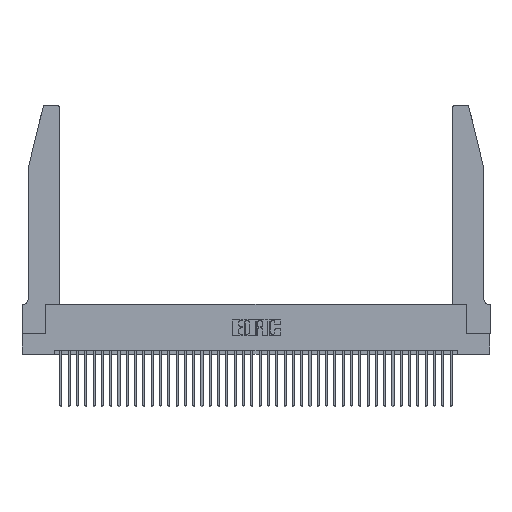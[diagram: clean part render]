
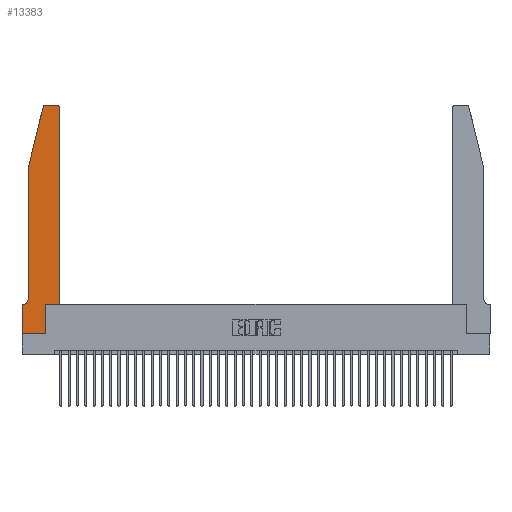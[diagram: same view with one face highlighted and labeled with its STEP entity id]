
A CAD part, top view. The second image highlights one B-rep face of the part: STEP entity #13383.
In plain terms, the highlighted planar face has unit normal (0, 0, 1).
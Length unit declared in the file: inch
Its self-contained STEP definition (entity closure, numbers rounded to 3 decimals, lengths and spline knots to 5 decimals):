
#378 = ORIENTED_EDGE ( 'NONE', *, *, #773, .T. ) ;
#773 = EDGE_CURVE ( 'NONE', #3050, #33618, #16278, .T. ) ;
#1754 = DIRECTION ( 'NONE',  ( -0.239, -0.971, 0. ) ) ;
#2519 = CARTESIAN_POINT ( 'NONE',  ( 0.0755, 2., 0.37 ) ) ;
#2624 = EDGE_CURVE ( 'NONE', #14654, #20736, #34224, .T. ) ;
#2860 = VERTEX_POINT ( 'NONE', #2519 ) ;
#3050 = VERTEX_POINT ( 'NONE', #29282 ) ;
#5523 = DIRECTION ( 'NONE',  ( 0., 0., 1. ) ) ;
#5721 = DIRECTION ( 'NONE',  ( 0., 0., 1. ) ) ;
#5935 = VERTEX_POINT ( 'NONE', #39529 ) ;
#6006 = AXIS2_PLACEMENT_3D ( 'NONE', #24862, #5721, #28077 ) ;
#6922 = ORIENTED_EDGE ( 'NONE', *, *, #25436, .T. ) ;
#7290 = CARTESIAN_POINT ( 'NONE',  ( 0.25487, 2.72718, 0.37 ) ) ;
#8300 = CARTESIAN_POINT ( 'NONE',  ( 0.4505, 0.35, 0.37 ) ) ;
#8853 = EDGE_CURVE ( 'NONE', #40166, #2860, #13556, .T. ) ;
#8968 = VERTEX_POINT ( 'NONE', #15034 ) ;
#9533 = CIRCLE ( 'NONE', #31428, 0.07 ) ;
#9796 = CARTESIAN_POINT ( 'NONE',  ( 0.2865, 0., 0.37 ) ) ;
#9949 = ORIENTED_EDGE ( 'NONE', *, *, #37876, .T. ) ;
#10384 = CARTESIAN_POINT ( 'NONE',  ( 0., 0., 0.37 ) ) ;
#10507 = FACE_OUTER_BOUND ( 'NONE', #39377, .T. ) ;
#10525 = DIRECTION ( 'NONE',  ( 0., 0., -1. ) ) ;
#10629 = CARTESIAN_POINT ( 'NONE',  ( 0.0055, 0.35, 0.37 ) ) ;
#10643 = DIRECTION ( 'NONE',  ( 1., 0., 0. ) ) ;
#10879 = VECTOR ( 'NONE', #37128, 39.37008 ) ;
#11299 = CARTESIAN_POINT ( 'NONE',  ( 0.2865, 0.35, 0.37 ) ) ;
#11422 = CARTESIAN_POINT ( 'NONE',  ( 0., 0., 0.37 ) ) ;
#11469 = ORIENTED_EDGE ( 'NONE', *, *, #29979, .T. ) ;
#12516 = AXIS2_PLACEMENT_3D ( 'NONE', #24664, #5523, #27863 ) ;
#13049 = VECTOR ( 'NONE', #33979, 39.37008 ) ;
#13055 = CIRCLE ( 'NONE', #6006, 0.03 ) ;
#13204 = VERTEX_POINT ( 'NONE', #24292 ) ;
#13383 = ADVANCED_FACE ( 'NONE', ( #10507 ), #31599, .T. ) ;
#13391 = VECTOR ( 'NONE', #10643, 39.37008 ) ;
#13556 = LINE ( 'NONE', #14614, #29543 ) ;
#14490 = ORIENTED_EDGE ( 'NONE', *, *, #14799, .T. ) ;
#14614 = CARTESIAN_POINT ( 'NONE',  ( 0.0755, 2., 0.37 ) ) ;
#14654 = VERTEX_POINT ( 'NONE', #9796 ) ;
#14799 = EDGE_CURVE ( 'NONE', #20736, #5935, #16878, .T. ) ;
#15034 = CARTESIAN_POINT ( 'NONE',  ( 0.284, 2.75, 0.37 ) ) ;
#16278 = CIRCLE ( 'NONE', #12516, 0.03 ) ;
#16878 = LINE ( 'NONE', #26118, #41525 ) ;
#16894 = CARTESIAN_POINT ( 'NONE',  ( 0.0755, 0.35, 0.37 ) ) ;
#17439 = ORIENTED_EDGE ( 'NONE', *, *, #27368, .T. ) ;
#17951 = CARTESIAN_POINT ( 'NONE',  ( 0.0755, 2., 0.37 ) ) ;
#18715 = AXIS2_PLACEMENT_3D ( 'NONE', #34753, #38128, #18847 ) ;
#18847 = DIRECTION ( 'NONE',  ( 1., 0., 0. ) ) ;
#19014 = CARTESIAN_POINT ( 'NONE',  ( 0.4205, 2.75, 0.37 ) ) ;
#20403 = EDGE_CURVE ( 'NONE', #5935, #3050, #34361, .T. ) ;
#20440 = ORIENTED_EDGE ( 'NONE', *, *, #38252, .T. ) ;
#20695 = VERTEX_POINT ( 'NONE', #22513 ) ;
#20736 = VERTEX_POINT ( 'NONE', #39027 ) ;
#21429 = DIRECTION ( 'NONE',  ( 0., 1., 0. ) ) ;
#21852 = LINE ( 'NONE', #32798, #13391 ) ;
#22513 = CARTESIAN_POINT ( 'NONE',  ( 0., 0.35, 0.37 ) ) ;
#23695 = VECTOR ( 'NONE', #30271, 39.37008 ) ;
#23969 = ORIENTED_EDGE ( 'NONE', *, *, #20403, .T. ) ;
#24292 = CARTESIAN_POINT ( 'NONE',  ( 0.0755, 0.42, 0.37 ) ) ;
#24664 = CARTESIAN_POINT ( 'NONE',  ( 0.4205, 2.72, 0.37 ) ) ;
#24691 = EDGE_CURVE ( 'NONE', #38850, #20695, #33551, .T. ) ;
#24707 = LINE ( 'NONE', #36674, #23695 ) ;
#24862 = CARTESIAN_POINT ( 'NONE',  ( 0.284, 2.72, 0.37 ) ) ;
#24958 = VECTOR ( 'NONE', #26517, 39.37008 ) ;
#25436 = EDGE_CURVE ( 'NONE', #33618, #8968, #24707, .T. ) ;
#25463 = ORIENTED_EDGE ( 'NONE', *, *, #24691, .T. ) ;
#25745 = VECTOR ( 'NONE', #21429, 39.37008 ) ;
#26118 = CARTESIAN_POINT ( 'NONE',  ( 0.4505, 0.35, 0.37 ) ) ;
#26517 = DIRECTION ( 'NONE',  ( -1., 0., 0. ) ) ;
#27368 = EDGE_CURVE ( 'NONE', #8968, #40166, #13055, .T. ) ;
#27863 = DIRECTION ( 'NONE',  ( 1., 0., 0. ) ) ;
#28077 = DIRECTION ( 'NONE',  ( 1., 0., 0. ) ) ;
#28466 = ORIENTED_EDGE ( 'NONE', *, *, #2624, .T. ) ;
#29282 = CARTESIAN_POINT ( 'NONE',  ( 0.4505, 2.72, 0.37 ) ) ;
#29543 = VECTOR ( 'NONE', #1754, 39.37008 ) ;
#29674 = CARTESIAN_POINT ( 'NONE',  ( 0.0055, 0.42, 0.37 ) ) ;
#29979 = EDGE_CURVE ( 'NONE', #31824, #14654, #21852, .T. ) ;
#30271 = DIRECTION ( 'NONE',  ( -1., 0., 0. ) ) ;
#30463 = DIRECTION ( 'NONE',  ( 0., 1., 0. ) ) ;
#31428 = AXIS2_PLACEMENT_3D ( 'NONE', #29674, #10525, #32946 ) ;
#31599 = PLANE ( 'NONE',  #18715 ) ;
#31824 = VERTEX_POINT ( 'NONE', #10384 ) ;
#32224 = EDGE_CURVE ( 'NONE', #20695, #31824, #37526, .T. ) ;
#32765 = DIRECTION ( 'NONE',  ( 1., 0., 0. ) ) ;
#32798 = CARTESIAN_POINT ( 'NONE',  ( 0., 0., 0.37 ) ) ;
#32946 = DIRECTION ( 'NONE',  ( -1., 0., 0. ) ) ;
#33200 = VECTOR ( 'NONE', #30463, 39.37008 ) ;
#33551 = LINE ( 'NONE', #16894, #24958 ) ;
#33618 = VERTEX_POINT ( 'NONE', #19014 ) ;
#33979 = DIRECTION ( 'NONE',  ( 0., -1., 0. ) ) ;
#34063 = ORIENTED_EDGE ( 'NONE', *, *, #32224, .T. ) ;
#34224 = LINE ( 'NONE', #11299, #33200 ) ;
#34361 = LINE ( 'NONE', #8300, #25745 ) ;
#34558 = ORIENTED_EDGE ( 'NONE', *, *, #8853, .T. ) ;
#34753 = CARTESIAN_POINT ( 'NONE',  ( 0., 0.35, 0.37 ) ) ;
#36674 = CARTESIAN_POINT ( 'NONE',  ( 0.2605, 2.75, 0.37 ) ) ;
#37128 = DIRECTION ( 'NONE',  ( 0., -1., 0. ) ) ;
#37526 = LINE ( 'NONE', #11422, #10879 ) ;
#37674 = LINE ( 'NONE', #17951, #13049 ) ;
#37876 = EDGE_CURVE ( 'NONE', #2860, #13204, #37674, .T. ) ;
#38128 = DIRECTION ( 'NONE',  ( 0., 0., 1. ) ) ;
#38252 = EDGE_CURVE ( 'NONE', #13204, #38850, #9533, .T. ) ;
#38850 = VERTEX_POINT ( 'NONE', #10629 ) ;
#39027 = CARTESIAN_POINT ( 'NONE',  ( 0.2865, 0.35, 0.37 ) ) ;
#39377 = EDGE_LOOP ( 'NONE', ( #6922, #17439, #34558, #9949, #20440, #25463, #34063, #11469, #28466, #14490, #23969, #378 ) ) ;
#39529 = CARTESIAN_POINT ( 'NONE',  ( 0.4505, 0.35, 0.37 ) ) ;
#40166 = VERTEX_POINT ( 'NONE', #7290 ) ;
#41525 = VECTOR ( 'NONE', #32765, 39.37008 ) ;
